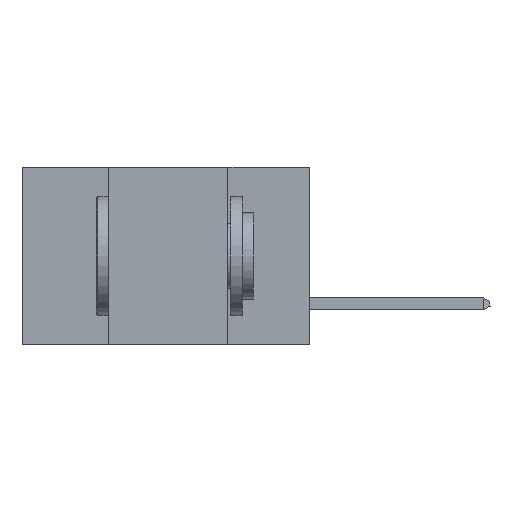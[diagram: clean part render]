
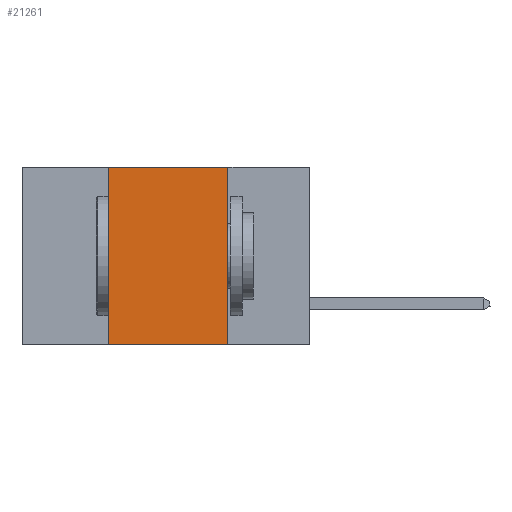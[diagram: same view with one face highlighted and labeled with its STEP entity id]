
A CAD part, left-side view. The second image highlights one B-rep face of the part: STEP entity #21261.
In plain terms, the highlighted planar face has unit normal (-1, 0, 0).
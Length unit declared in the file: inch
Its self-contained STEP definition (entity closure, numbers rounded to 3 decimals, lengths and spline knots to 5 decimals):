
#257 = ORIENTED_EDGE ( 'NONE', *, *, #13011, .T. ) ;
#1817 = FACE_OUTER_BOUND ( 'NONE', #18917, .T. ) ;
#3019 = EDGE_CURVE ( 'NONE', #8139, #36091, #30727, .T. ) ;
#4253 = DIRECTION ( 'NONE',  ( 0., 0., -1. ) ) ;
#4716 = CARTESIAN_POINT ( 'NONE',  ( 0., 0.17, 0. ) ) ;
#5675 = LINE ( 'NONE', #21819, #24668 ) ;
#6593 = VECTOR ( 'NONE', #10532, 39.37008 ) ;
#7193 = CARTESIAN_POINT ( 'NONE',  ( 0., 0.17, -0.37 ) ) ;
#7845 = DIRECTION ( 'NONE',  ( 0., 0., 1. ) ) ;
#8139 = VERTEX_POINT ( 'NONE', #11691 ) ;
#10093 = PLANE ( 'NONE',  #27452 ) ;
#10532 = DIRECTION ( 'NONE',  ( 0., 0., -1. ) ) ;
#11466 = VERTEX_POINT ( 'NONE', #21157 ) ;
#11624 = VECTOR ( 'NONE', #7845, 39.37008 ) ;
#11691 = CARTESIAN_POINT ( 'NONE',  ( 0., 0.17, 0. ) ) ;
#12536 = LINE ( 'NONE', #33755, #11624 ) ;
#12808 = CARTESIAN_POINT ( 'NONE',  ( 0., 0.6, 0. ) ) ;
#13011 = EDGE_CURVE ( 'NONE', #15453, #36091, #33315, .T. ) ;
#15039 = ORIENTED_EDGE ( 'NONE', *, *, #3019, .F. ) ;
#15304 = EDGE_CURVE ( 'NONE', #11466, #8139, #5675, .T. ) ;
#15429 = DIRECTION ( 'NONE',  ( 0., -1., 0. ) ) ;
#15453 = VERTEX_POINT ( 'NONE', #29756 ) ;
#15633 = EDGE_CURVE ( 'NONE', #15453, #11466, #12536, .T. ) ;
#18917 = EDGE_LOOP ( 'NONE', ( #15039, #29898, #21566, #257 ) ) ;
#21157 = CARTESIAN_POINT ( 'NONE',  ( 0., 0.42, 0. ) ) ;
#21261 = ADVANCED_FACE ( 'NONE', ( #1817 ), #10093, .F. ) ;
#21566 = ORIENTED_EDGE ( 'NONE', *, *, #15633, .F. ) ;
#21819 = CARTESIAN_POINT ( 'NONE',  ( 0., 0.6, 0. ) ) ;
#24193 = CARTESIAN_POINT ( 'NONE',  ( 0., 0.6, -0.37 ) ) ;
#24668 = VECTOR ( 'NONE', #36596, 39.37008 ) ;
#25041 = DIRECTION ( 'NONE',  ( 1., 0., 0. ) ) ;
#27452 = AXIS2_PLACEMENT_3D ( 'NONE', #12808, #25041, #4253 ) ;
#29756 = CARTESIAN_POINT ( 'NONE',  ( 0., 0.42, -0.37 ) ) ;
#29898 = ORIENTED_EDGE ( 'NONE', *, *, #15304, .F. ) ;
#30727 = LINE ( 'NONE', #4716, #6593 ) ;
#33315 = LINE ( 'NONE', #24193, #35662 ) ;
#33755 = CARTESIAN_POINT ( 'NONE',  ( 0., 0.42, 0. ) ) ;
#35662 = VECTOR ( 'NONE', #15429, 39.37008 ) ;
#36091 = VERTEX_POINT ( 'NONE', #7193 ) ;
#36596 = DIRECTION ( 'NONE',  ( 0., -1., 0. ) ) ;
